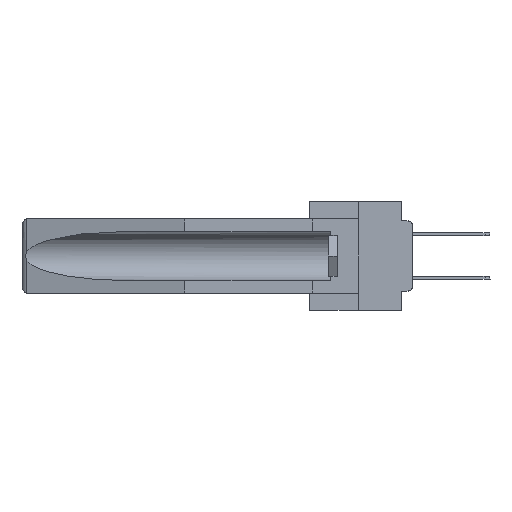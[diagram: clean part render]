
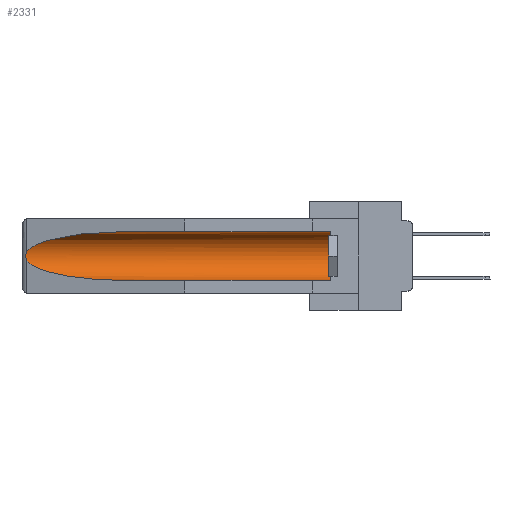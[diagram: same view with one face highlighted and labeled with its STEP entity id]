
A CAD part, left-side view. The second image highlights one B-rep face of the part: STEP entity #2331.
In plain terms, the highlighted cylindrical face has radius 2.857 mm (diameter 5.715 mm), a partial arc.
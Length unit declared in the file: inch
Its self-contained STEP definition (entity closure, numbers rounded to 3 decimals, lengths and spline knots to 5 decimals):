
#413 = VERTEX_POINT ( 'NONE', #3014 ) ;
#1089 = CARTESIAN_POINT ( 'NONE',  ( 0.155, 0.126, -0.284 ) ) ;
#1214 = ORIENTED_EDGE ( 'NONE', *, *, #10810, .F. ) ;
#1449 = CARTESIAN_POINT ( 'NONE',  ( 0.155, -0.30754, -0.1715 ) ) ;
#1550 = CARTESIAN_POINT ( 'NONE',  ( 0.155, 1.07973, -0.059 ) ) ;
#2331 = ADVANCED_FACE ( 'NONE', ( #17007 ), #21837, .F. ) ;
#3014 = CARTESIAN_POINT ( 'NONE',  ( 0.155, 1.07973, -0.284 ) ) ;
#3217 = VERTEX_POINT ( 'NONE', #12261 ) ;
#3305 = ORIENTED_EDGE ( 'NONE', *, *, #23012, .T. ) ;
#3641 = ORIENTED_EDGE ( 'NONE', *, *, #16067, .T. ) ;
#4051 = DIRECTION ( 'NONE',  ( 0., 1., 0. ) ) ;
#4098 = EDGE_CURVE ( 'NONE', #3217, #7415, #10227, .T. ) ;
#4684 = CIRCLE ( 'NONE', #26407, 0.1125 ) ;
#5624 = CARTESIAN_POINT ( 'NONE',  ( 0.155, 0.126, -0.1715 ) ) ;
#5714 = CARTESIAN_POINT ( 'NONE',  ( 0.155, -0.30754, -0.059 ) ) ;
#5734 = CARTESIAN_POINT ( 'NONE',  ( 0.26537, 1.52718, -0.14972 ) ) ;
#5885 = CARTESIAN_POINT ( 'NONE',  ( 0.26597, 1.52961, -0.15275 ) ) ;
#6959 = CARTESIAN_POINT ( 'NONE',  ( 0.21114, 1.30732, -0.284 ) ) ;
#7204 = ORIENTED_EDGE ( 'NONE', *, *, #24372, .T. ) ;
#7415 = VERTEX_POINT ( 'NONE', #1550 ) ;
#7882 = CARTESIAN_POINT ( 'NONE',  ( 0.26537, 1.52718, -0.19328 ) ) ;
#8172 = DIRECTION ( 'NONE',  ( 0., 0., 1. ) ) ;
#10184 = CARTESIAN_POINT ( 'NONE',  ( 0.21114, 1.30732, -0.059 ) ) ;
#10227 = LINE ( 'NONE', #5714, #20779 ) ;
#10810 = EDGE_CURVE ( 'NONE', #25651, #413, #11145, .T. ) ;
#11145 = LINE ( 'NONE', #29573, #19714 ) ;
#11541 = CARTESIAN_POINT ( 'NONE',  ( 0.26537, 1.52718, -0.14972 ) ) ;
#12261 = CARTESIAN_POINT ( 'NONE',  ( 0.155, 0.126, -0.059 ) ) ;
#13406 = CARTESIAN_POINT ( 'NONE',  ( 0.26537, 1.52718, -0.19328 ) ) ;
#13747 = CARTESIAN_POINT ( 'NONE',  ( 0.25451, 1.48313, -0.24835 ) ) ;
#14937 = CARTESIAN_POINT ( 'NONE',  ( 0.2673, 1.5327, -0.16383 ) ) ;
#16067 = EDGE_CURVE ( 'NONE', #17067, #413, #20125, .T. ) ;
#16315 = CARTESIAN_POINT ( 'NONE',  ( 0.155, 1.07973, -0.284 ) ) ;
#17007 = FACE_OUTER_BOUND ( 'NONE', #19668, .T. ) ;
#17067 = VERTEX_POINT ( 'NONE', #7882 ) ;
#17331 = CARTESIAN_POINT ( 'NONE',  ( 0.2673, 1.53269, -0.17917 ) ) ;
#17776 = CARTESIAN_POINT ( 'NONE',  ( 0.26597, 1.5296, -0.19026 ) ) ;
#18811 = ORIENTED_EDGE ( 'NONE', *, *, #4098, .T. ) ;
#19381 = CARTESIAN_POINT ( 'NONE',  ( 0.25451, 1.48313, -0.09465 ) ) ;
#19595 = CARTESIAN_POINT ( 'NONE',  ( 0.26654, 1.53092, -0.15636 ) ) ;
#19668 = EDGE_LOOP ( 'NONE', ( #25939, #3305, #3641, #1214, #7204, #18811 ) ) ;
#19714 = VECTOR ( 'NONE', #4051, 39.37008 ) ;
#19897 =( BOUNDED_CURVE ( )  B_SPLINE_CURVE ( 3, ( #21647, #10184, #19381, #26353 ),
 .UNSPECIFIED., .F., .F. ) 
 B_SPLINE_CURVE_WITH_KNOTS ( ( 4, 4 ),
 ( 4.71239, 6.08839 ),
 .UNSPECIFIED. ) 
 CURVE ( )  GEOMETRIC_REPRESENTATION_ITEM ( )  RATIONAL_B_SPLINE_CURVE ( ( 1., 0.848, 0.848, 1. ) ) 
 REPRESENTATION_ITEM ( '' )  );
#20125 =( BOUNDED_CURVE ( )  B_SPLINE_CURVE ( 3, ( #20673, #13747, #6959, #16315 ),
 .UNSPECIFIED., .F., .F. ) 
 B_SPLINE_CURVE_WITH_KNOTS ( ( 4, 4 ),
 ( 0.1948, 1.5708 ),
 .UNSPECIFIED. ) 
 CURVE ( )  GEOMETRIC_REPRESENTATION_ITEM ( )  RATIONAL_B_SPLINE_CURVE ( ( 1., 0.848, 0.848, 1. ) ) 
 REPRESENTATION_ITEM ( '' )  );
#20673 = CARTESIAN_POINT ( 'NONE',  ( 0.26537, 1.52718, -0.19328 ) ) ;
#20779 = VECTOR ( 'NONE', #23668, 39.37008 ) ;
#21647 = CARTESIAN_POINT ( 'NONE',  ( 0.155, 1.07973, -0.059 ) ) ;
#21837 = CYLINDRICAL_SURFACE ( 'NONE', #22486, 0.1125 ) ;
#22133 = DIRECTION ( 'NONE',  ( 0., 0., 1. ) ) ;
#22486 = AXIS2_PLACEMENT_3D ( 'NONE', #1449, #26390, #22133 ) ;
#23012 = EDGE_CURVE ( 'NONE', #27751, #17067, #29071, .T. ) ;
#23668 = DIRECTION ( 'NONE',  ( 0., 1., 0. ) ) ;
#24029 = DIRECTION ( 'NONE',  ( 0., -1., 0. ) ) ;
#24132 = CARTESIAN_POINT ( 'NONE',  ( 0.2675, 1.53308, -0.16763 ) ) ;
#24372 = EDGE_CURVE ( 'NONE', #25651, #3217, #4684, .T. ) ;
#25233 = EDGE_CURVE ( 'NONE', #7415, #27751, #19897, .T. ) ;
#25651 = VERTEX_POINT ( 'NONE', #1089 ) ;
#25939 = ORIENTED_EDGE ( 'NONE', *, *, #25233, .T. ) ;
#26353 = CARTESIAN_POINT ( 'NONE',  ( 0.26537, 1.52718, -0.14972 ) ) ;
#26390 = DIRECTION ( 'NONE',  ( 0., 1., 0. ) ) ;
#26407 = AXIS2_PLACEMENT_3D ( 'NONE', #5624, #24029, #8172 ) ;
#26570 = CARTESIAN_POINT ( 'NONE',  ( 0.26655, 1.53094, -0.18657 ) ) ;
#27751 = VERTEX_POINT ( 'NONE', #11541 ) ;
#28823 = CARTESIAN_POINT ( 'NONE',  ( 0.2675, 1.53308, -0.17534 ) ) ;
#29071 = B_SPLINE_CURVE_WITH_KNOTS ( 'NONE', 3,
 ( #5734, #5885, #19595, #14937, #24132, #28823, #17331, #26570, #17776, #13406 ),
 .UNSPECIFIED., .F., .F.,
 ( 4, 2, 2, 2, 4 ),
 ( 0., 0.00029, 0.00058, 0.00087, 0.00117 ),
 .UNSPECIFIED. ) ;
#29573 = CARTESIAN_POINT ( 'NONE',  ( 0.155, -0.30754, -0.284 ) ) ;
